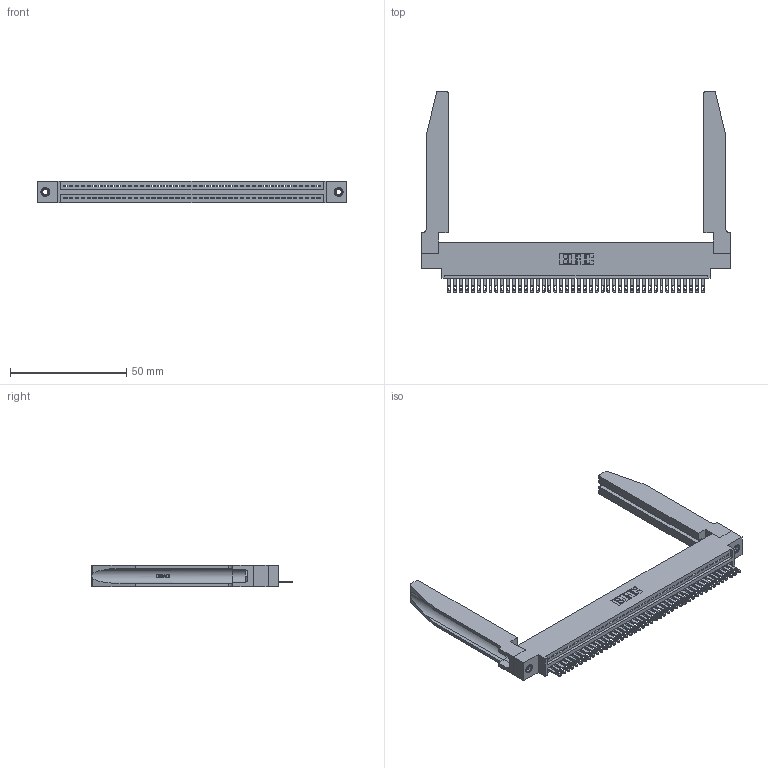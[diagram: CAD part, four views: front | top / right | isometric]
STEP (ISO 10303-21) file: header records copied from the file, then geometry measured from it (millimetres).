
FILE_DESCRIPTION (( 'STEP AP203' ), '1' );
FILE_NAME ('345-044-500-678.STEP', '2019-10-08T18:10:21', ( '' ), ( '' ), 'SwSTEP 2.0', 'SolidWorks 2016', '' );
FILE_SCHEMA (( 'CONFIG_CONTROL_DESIGN' ));
Length unit declared in the file: inch
Products named in the file (5): 345 Part_0.170 Offset - 0.156 Dia-TH; 345-292-001_345-293-100; 345-044-500-678; 345-220-078_345-220-078; 345-250-001_345-250-001-102
Assembly tree (49 placements, depth 2):
  345-044-500-678
    345 Part_0.170 Offset - 0.156 Dia-TH
    345-292-001_345-293-100  x44
    345-250-001_345-250-001-102  x2
    345-220-078_345-220-078  x2
Bounding box: 132.99 x 86.79 x 9.4 mm (x, y, z)
Volume: 20332.7 mm3; surface area: 23792.1 mm2
Topology: 49 solids, 49 shells, 2740 faces, 8353 edges, 5558 vertices
Faces by surface type: plane 1722, cylinder 966, bspline 36, cone 12, torus 4
Entity records: 37648 total; most frequent: CARTESIAN_POINT 7419, ORIENTED_EDGE 6294, DIRECTION 5485, EDGE_CURVE 3147, VECTOR 2741, LINE 2741, VERTEX_POINT 2092, AXIS2_PLACEMENT_3D 1372
